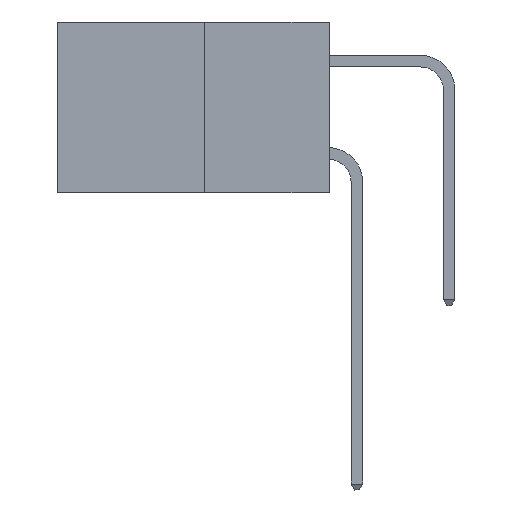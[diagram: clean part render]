
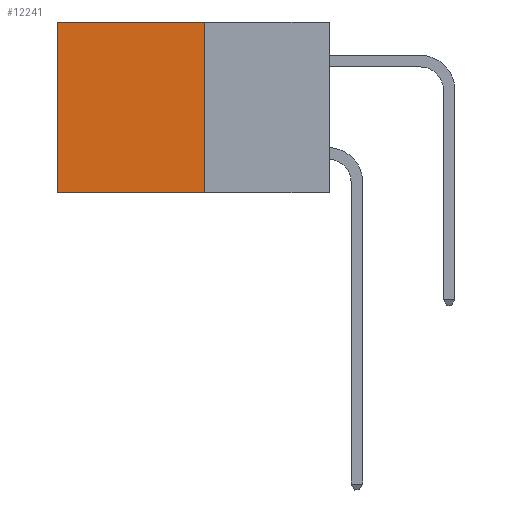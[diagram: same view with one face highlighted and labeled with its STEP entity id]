
A CAD part, left-side view. The second image highlights one B-rep face of the part: STEP entity #12241.
In plain terms, the highlighted planar face has unit normal (-1, 0, 0).
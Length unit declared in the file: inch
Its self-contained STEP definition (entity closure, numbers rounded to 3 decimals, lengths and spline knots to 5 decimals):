
#222 = CARTESIAN_POINT ( 'NONE',  ( 0.277, 0.59, -0.37 ) ) ;
#514 = CARTESIAN_POINT ( 'NONE',  ( 0.277, 0.27, -0.37 ) ) ;
#1818 = EDGE_CURVE ( 'NONE', #7334, #4540, #24817, .T. ) ;
#2402 = VERTEX_POINT ( 'NONE', #7896 ) ;
#3793 = VECTOR ( 'NONE', #4744, 39.37008 ) ;
#4174 = CARTESIAN_POINT ( 'NONE',  ( 0.277, 0.27, 0. ) ) ;
#4472 = LINE ( 'NONE', #4174, #3793 ) ;
#4540 = VERTEX_POINT ( 'NONE', #18793 ) ;
#4744 = DIRECTION ( 'NONE',  ( 0., 1., 0. ) ) ;
#5075 = ORIENTED_EDGE ( 'NONE', *, *, #10149, .F. ) ;
#5624 = EDGE_CURVE ( 'NONE', #2402, #7334, #4472, .T. ) ;
#6173 = ORIENTED_EDGE ( 'NONE', *, *, #1818, .T. ) ;
#6915 = ORIENTED_EDGE ( 'NONE', *, *, #5624, .T. ) ;
#7334 = VERTEX_POINT ( 'NONE', #23471 ) ;
#7896 = CARTESIAN_POINT ( 'NONE',  ( 0.277, 0.27, 0. ) ) ;
#8214 = EDGE_LOOP ( 'NONE', ( #6173, #11576, #5075, #6915 ) ) ;
#10149 = EDGE_CURVE ( 'NONE', #2402, #18791, #18951, .T. ) ;
#10703 = DIRECTION ( 'NONE',  ( 1., 0., 0. ) ) ;
#11576 = ORIENTED_EDGE ( 'NONE', *, *, #17520, .F. ) ;
#12241 = ADVANCED_FACE ( 'NONE', ( #16612 ), #22534, .F. ) ;
#12258 = CARTESIAN_POINT ( 'NONE',  ( 0.277, 0.27, -0.37 ) ) ;
#13764 = VECTOR ( 'NONE', #14760, 39.37008 ) ;
#13850 = LINE ( 'NONE', #14120, #18558 ) ;
#14120 = CARTESIAN_POINT ( 'NONE',  ( 0.277, 0.27, -0.37 ) ) ;
#14265 = DIRECTION ( 'NONE',  ( 0., 0., -1. ) ) ;
#14760 = DIRECTION ( 'NONE',  ( 0., 0., -1. ) ) ;
#15699 = CARTESIAN_POINT ( 'NONE',  ( 0.277, 0.27, -0.37 ) ) ;
#16612 = FACE_OUTER_BOUND ( 'NONE', #8214, .T. ) ;
#17520 = EDGE_CURVE ( 'NONE', #18791, #4540, #13850, .T. ) ;
#18321 = VECTOR ( 'NONE', #14265, 39.37008 ) ;
#18558 = VECTOR ( 'NONE', #20150, 39.37008 ) ;
#18791 = VERTEX_POINT ( 'NONE', #15699 ) ;
#18793 = CARTESIAN_POINT ( 'NONE',  ( 0.277, 0.59, -0.37 ) ) ;
#18951 = LINE ( 'NONE', #12258, #18321 ) ;
#20150 = DIRECTION ( 'NONE',  ( 0., 1., 0. ) ) ;
#20681 = AXIS2_PLACEMENT_3D ( 'NONE', #514, #10703, #24453 ) ;
#22534 = PLANE ( 'NONE',  #20681 ) ;
#23471 = CARTESIAN_POINT ( 'NONE',  ( 0.277, 0.59, 0. ) ) ;
#24453 = DIRECTION ( 'NONE',  ( 0., 0., -1. ) ) ;
#24817 = LINE ( 'NONE', #222, #13764 ) ;
